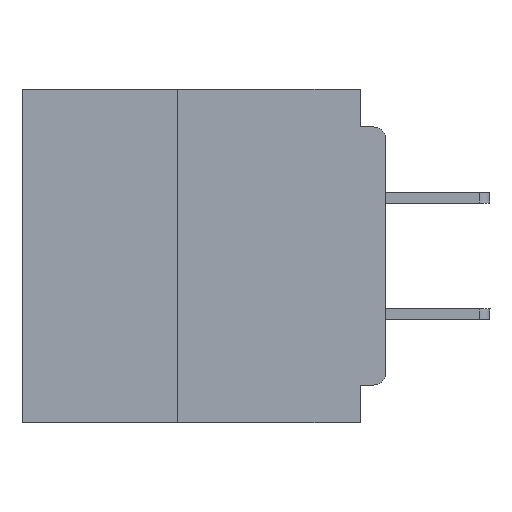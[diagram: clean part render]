
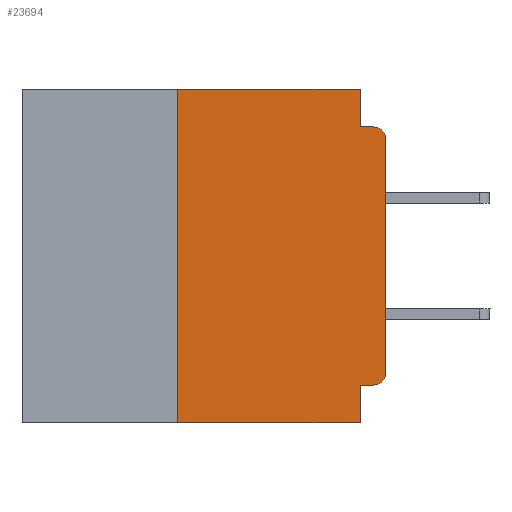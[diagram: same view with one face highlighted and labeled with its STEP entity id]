
A CAD part, left-side view. The second image highlights one B-rep face of the part: STEP entity #23694.
In plain terms, the highlighted planar face has unit normal (-1, 0, 0).
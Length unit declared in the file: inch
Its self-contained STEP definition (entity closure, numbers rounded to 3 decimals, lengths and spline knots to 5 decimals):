
#660 = EDGE_CURVE ( 'NONE', #45743, #62114, #16503, .T. ) ;
#921 = DIRECTION ( 'NONE',  ( 0., 0., -1. ) ) ;
#1897 = ORIENTED_EDGE ( 'NONE', *, *, #34662, .T. ) ;
#2632 = VERTEX_POINT ( 'NONE', #15319 ) ;
#2796 = CARTESIAN_POINT ( 'NONE',  ( 0., 0.015, -0.045 ) ) ;
#3828 = VERTEX_POINT ( 'NONE', #40176 ) ;
#3968 = CARTESIAN_POINT ( 'NONE',  ( 0., 0., 0. ) ) ;
#4401 = AXIS2_PLACEMENT_3D ( 'NONE', #58315, #28972, #63246 ) ;
#4427 = EDGE_CURVE ( 'NONE', #46580, #2632, #42251, .T. ) ;
#5944 = VERTEX_POINT ( 'NONE', #52384 ) ;
#7453 = CARTESIAN_POINT ( 'NONE',  ( 0., 0.031, 0. ) ) ;
#7642 = CARTESIAN_POINT ( 'NONE',  ( 0., 0.437, -0.4 ) ) ;
#8932 = EDGE_CURVE ( 'NONE', #46580, #3828, #62825, .T. ) ;
#9182 = DIRECTION ( 'NONE',  ( 0., 0., 1. ) ) ;
#9484 = DIRECTION ( 'NONE',  ( 0., 0., 1. ) ) ;
#10766 = VECTOR ( 'NONE', #39471, 39.37008 ) ;
#11122 = LINE ( 'NONE', #7642, #34262 ) ;
#12922 = ORIENTED_EDGE ( 'NONE', *, *, #35103, .T. ) ;
#13647 = ORIENTED_EDGE ( 'NONE', *, *, #4427, .F. ) ;
#14666 = ORIENTED_EDGE ( 'NONE', *, *, #660, .F. ) ;
#15319 = CARTESIAN_POINT ( 'NONE',  ( 0., 0.031, -0.355 ) ) ;
#16503 = LINE ( 'NONE', #22435, #54159 ) ;
#17122 = LINE ( 'NONE', #3968, #54783 ) ;
#17746 = PLANE ( 'NONE',  #36804 ) ;
#17872 = CARTESIAN_POINT ( 'NONE',  ( 0., 0., -0.045 ) ) ;
#17939 = EDGE_CURVE ( 'NONE', #2632, #5944, #35179, .T. ) ;
#20808 = FACE_OUTER_BOUND ( 'NONE', #37445, .T. ) ;
#21040 = ORIENTED_EDGE ( 'NONE', *, *, #50635, .F. ) ;
#22435 = CARTESIAN_POINT ( 'NONE',  ( 0., 0.25, -0.4 ) ) ;
#22548 = EDGE_CURVE ( 'NONE', #59636, #47639, #30727, .T. ) ;
#22700 = DIRECTION ( 'NONE',  ( -1., 0., 0. ) ) ;
#22717 = DIRECTION ( 'NONE',  ( 1., 0., 0. ) ) ;
#23694 = ADVANCED_FACE ( 'NONE', ( #20808 ), #17746, .F. ) ;
#24168 = DIRECTION ( 'NONE',  ( 0., 0., -1. ) ) ;
#24811 = CARTESIAN_POINT ( 'NONE',  ( 0., 0.25, 0. ) ) ;
#25323 = VERTEX_POINT ( 'NONE', #7453 ) ;
#25701 = CARTESIAN_POINT ( 'NONE',  ( 0., 0.031, 0. ) ) ;
#26142 = VERTEX_POINT ( 'NONE', #29491 ) ;
#28972 = DIRECTION ( 'NONE',  ( -1., 0., 0. ) ) ;
#29491 = CARTESIAN_POINT ( 'NONE',  ( 0., 0., -0.06 ) ) ;
#30727 = LINE ( 'NONE', #17872, #55267 ) ;
#33630 = VECTOR ( 'NONE', #24168, 39.37008 ) ;
#34262 = VECTOR ( 'NONE', #42176, 39.37008 ) ;
#34455 = CARTESIAN_POINT ( 'NONE',  ( 0., 0.015, -0.355 ) ) ;
#34487 = ORIENTED_EDGE ( 'NONE', *, *, #17939, .F. ) ;
#34662 = EDGE_CURVE ( 'NONE', #26142, #47639, #47352, .T. ) ;
#35103 = EDGE_CURVE ( 'NONE', #45743, #5944, #11122, .T. ) ;
#35179 = LINE ( 'NONE', #63429, #33630 ) ;
#35627 = CARTESIAN_POINT ( 'NONE',  ( 0., 0., -0.355 ) ) ;
#36196 = ORIENTED_EDGE ( 'NONE', *, *, #22548, .F. ) ;
#36804 = AXIS2_PLACEMENT_3D ( 'NONE', #61789, #22717, #57055 ) ;
#37047 = LINE ( 'NONE', #49097, #10766 ) ;
#37443 = CARTESIAN_POINT ( 'NONE',  ( 0., 0.031, -0.045 ) ) ;
#37445 = EDGE_LOOP ( 'NONE', ( #50191, #1897, #36196, #43159, #21040, #14666, #12922, #34487, #13647, #49342 ) ) ;
#39471 = DIRECTION ( 'NONE',  ( 0., -1., 0. ) ) ;
#39547 = EDGE_CURVE ( 'NONE', #3828, #26142, #17122, .T. ) ;
#40176 = CARTESIAN_POINT ( 'NONE',  ( 0., 0., -0.34 ) ) ;
#42176 = DIRECTION ( 'NONE',  ( 0., -1., 0. ) ) ;
#42251 = LINE ( 'NONE', #35627, #53752 ) ;
#43159 = ORIENTED_EDGE ( 'NONE', *, *, #61177, .F. ) ;
#45743 = VERTEX_POINT ( 'NONE', #51925 ) ;
#46495 = VECTOR ( 'NONE', #921, 39.37008 ) ;
#46580 = VERTEX_POINT ( 'NONE', #34455 ) ;
#47352 = CIRCLE ( 'NONE', #4401, 0.015 ) ;
#47639 = VERTEX_POINT ( 'NONE', #2796 ) ;
#49097 = CARTESIAN_POINT ( 'NONE',  ( 0., 0.437, 0. ) ) ;
#49342 = ORIENTED_EDGE ( 'NONE', *, *, #8932, .T. ) ;
#49418 = AXIS2_PLACEMENT_3D ( 'NONE', #52129, #22700, #57041 ) ;
#50191 = ORIENTED_EDGE ( 'NONE', *, *, #39547, .T. ) ;
#50197 = DIRECTION ( 'NONE',  ( 0., 1., 0. ) ) ;
#50635 = EDGE_CURVE ( 'NONE', #62114, #25323, #37047, .T. ) ;
#51925 = CARTESIAN_POINT ( 'NONE',  ( 0., 0.25, -0.4 ) ) ;
#52129 = CARTESIAN_POINT ( 'NONE',  ( 0., 0.015, -0.34 ) ) ;
#52384 = CARTESIAN_POINT ( 'NONE',  ( 0., 0.031, -0.4 ) ) ;
#53752 = VECTOR ( 'NONE', #50197, 39.37008 ) ;
#54159 = VECTOR ( 'NONE', #9484, 39.37008 ) ;
#54783 = VECTOR ( 'NONE', #9182, 39.37008 ) ;
#55267 = VECTOR ( 'NONE', #61906, 39.37008 ) ;
#57041 = DIRECTION ( 'NONE',  ( 0., 0., -1. ) ) ;
#57055 = DIRECTION ( 'NONE',  ( 0., 0., -1. ) ) ;
#58315 = CARTESIAN_POINT ( 'NONE',  ( 0., 0.015, -0.06 ) ) ;
#59636 = VERTEX_POINT ( 'NONE', #37443 ) ;
#61177 = EDGE_CURVE ( 'NONE', #25323, #59636, #62621, .T. ) ;
#61789 = CARTESIAN_POINT ( 'NONE',  ( 0., 0.437, 0. ) ) ;
#61906 = DIRECTION ( 'NONE',  ( 0., -1., 0. ) ) ;
#62114 = VERTEX_POINT ( 'NONE', #24811 ) ;
#62621 = LINE ( 'NONE', #25701, #46495 ) ;
#62825 = CIRCLE ( 'NONE', #49418, 0.015 ) ;
#63246 = DIRECTION ( 'NONE',  ( 0., 0., -1. ) ) ;
#63429 = CARTESIAN_POINT ( 'NONE',  ( 0., 0.031, -0.4 ) ) ;
